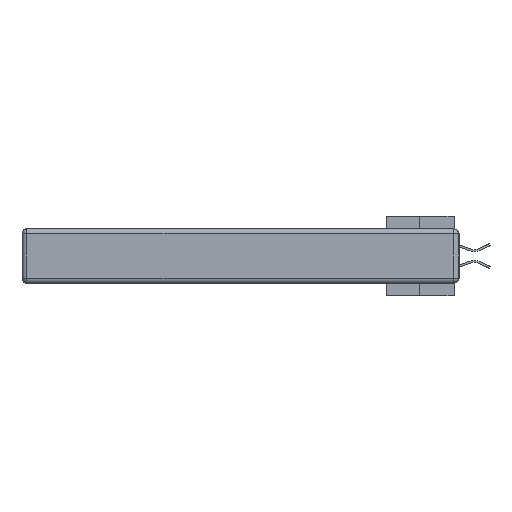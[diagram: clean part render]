
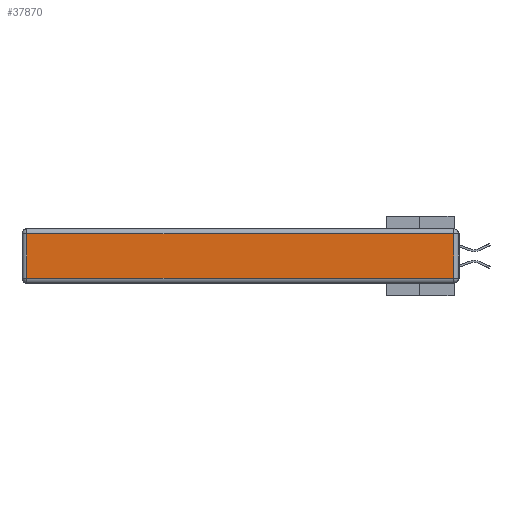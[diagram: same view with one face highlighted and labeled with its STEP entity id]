
A CAD part, left-side view. The second image highlights one B-rep face of the part: STEP entity #37870.
In plain terms, the highlighted planar face has unit normal (-1, 0, 0).
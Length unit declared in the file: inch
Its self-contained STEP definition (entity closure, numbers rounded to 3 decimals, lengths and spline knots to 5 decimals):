
#3128 = CARTESIAN_POINT ( 'NONE',  ( 0., 0.03, -0.03 ) ) ;
#3641 = CARTESIAN_POINT ( 'NONE',  ( 0., 2.72, -0.313 ) ) ;
#4132 = VERTEX_POINT ( 'NONE', #3641 ) ;
#4703 = VECTOR ( 'NONE', #28268, 39.37008 ) ;
#4856 = VECTOR ( 'NONE', #23719, 39.37008 ) ;
#8070 = CARTESIAN_POINT ( 'NONE',  ( 0., 0., -0.313 ) ) ;
#8280 = EDGE_CURVE ( 'NONE', #33782, #8512, #20792, .T. ) ;
#8512 = VERTEX_POINT ( 'NONE', #3128 ) ;
#8518 = LINE ( 'NONE', #49030, #20398 ) ;
#8735 = CARTESIAN_POINT ( 'NONE',  ( 0., 2.75, -0.03 ) ) ;
#14354 = ORIENTED_EDGE ( 'NONE', *, *, #8280, .T. ) ;
#15842 = CARTESIAN_POINT ( 'NONE',  ( 0., 0., -0.343 ) ) ;
#16484 = PLANE ( 'NONE',  #29277 ) ;
#16621 = CARTESIAN_POINT ( 'NONE',  ( 0., 2.72, -0.03 ) ) ;
#16692 = EDGE_CURVE ( 'NONE', #8512, #31553, #30488, .T. ) ;
#17926 = FACE_OUTER_BOUND ( 'NONE', #36808, .T. ) ;
#19807 = DIRECTION ( 'NONE',  ( 0., 0., 1. ) ) ;
#20398 = VECTOR ( 'NONE', #26128, 39.37008 ) ;
#20792 = LINE ( 'NONE', #38394, #4703 ) ;
#21290 = LINE ( 'NONE', #8070, #46437 ) ;
#22400 = EDGE_CURVE ( 'NONE', #4132, #33782, #21290, .T. ) ;
#23719 = DIRECTION ( 'NONE',  ( 0., 1., 0. ) ) ;
#26128 = DIRECTION ( 'NONE',  ( 0., 0., -1. ) ) ;
#28268 = DIRECTION ( 'NONE',  ( 0., 0., 1. ) ) ;
#29277 = AXIS2_PLACEMENT_3D ( 'NONE', #15842, #38866, #19807 ) ;
#29329 = ORIENTED_EDGE ( 'NONE', *, *, #22400, .T. ) ;
#30488 = LINE ( 'NONE', #8735, #4856 ) ;
#31173 = ORIENTED_EDGE ( 'NONE', *, *, #49312, .T. ) ;
#31553 = VERTEX_POINT ( 'NONE', #16621 ) ;
#32358 = ORIENTED_EDGE ( 'NONE', *, *, #16692, .T. ) ;
#33782 = VERTEX_POINT ( 'NONE', #35266 ) ;
#35140 = DIRECTION ( 'NONE',  ( 0., -1., 0. ) ) ;
#35266 = CARTESIAN_POINT ( 'NONE',  ( 0., 0.03, -0.313 ) ) ;
#36808 = EDGE_LOOP ( 'NONE', ( #29329, #14354, #32358, #31173 ) ) ;
#37870 = ADVANCED_FACE ( 'NONE', ( #17926 ), #16484, .T. ) ;
#38394 = CARTESIAN_POINT ( 'NONE',  ( 0., 0.03, -0.343 ) ) ;
#38866 = DIRECTION ( 'NONE',  ( -1., 0., 0. ) ) ;
#46437 = VECTOR ( 'NONE', #35140, 39.37008 ) ;
#49030 = CARTESIAN_POINT ( 'NONE',  ( 0., 2.72, -0.343 ) ) ;
#49312 = EDGE_CURVE ( 'NONE', #31553, #4132, #8518, .T. ) ;
